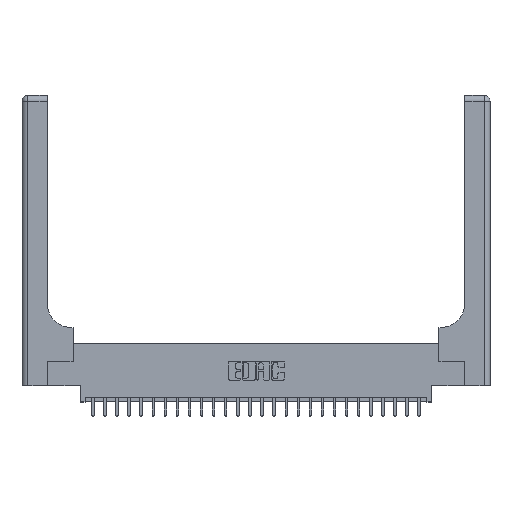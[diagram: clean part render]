
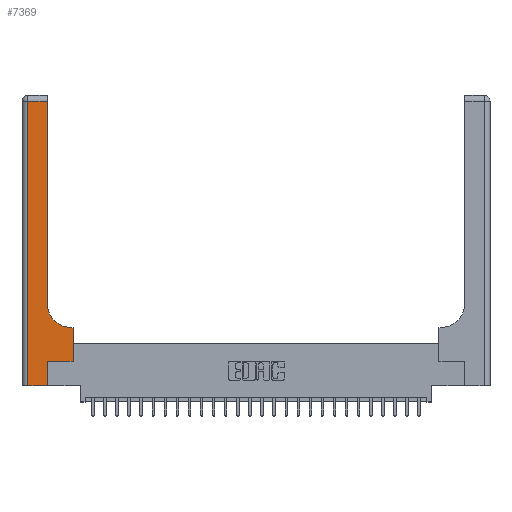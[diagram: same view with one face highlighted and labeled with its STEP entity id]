
A CAD part, top view. The second image highlights one B-rep face of the part: STEP entity #7369.
In plain terms, the highlighted planar face has unit normal (0, 0, 1).
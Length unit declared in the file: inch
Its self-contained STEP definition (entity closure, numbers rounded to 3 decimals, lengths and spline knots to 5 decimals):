
#612 = CARTESIAN_POINT ( 'NONE',  ( 0.26, 2.94, 0.37 ) ) ;
#1178 = LINE ( 'NONE', #20961, #21587 ) ;
#1230 = DIRECTION ( 'NONE',  ( 0., 1., 0. ) ) ;
#1351 = ORIENTED_EDGE ( 'NONE', *, *, #3178, .T. ) ;
#1502 = CARTESIAN_POINT ( 'NONE',  ( 0.265, 0., 0.37 ) ) ;
#1601 = LINE ( 'NONE', #24904, #11589 ) ;
#1966 = CARTESIAN_POINT ( 'NONE',  ( 0., 3., 0.37 ) ) ;
#2355 = CARTESIAN_POINT ( 'NONE',  ( 0.265, 0.25, 0.37 ) ) ;
#3028 = CARTESIAN_POINT ( 'NONE',  ( 0.51, 0.85, 0.37 ) ) ;
#3178 = EDGE_CURVE ( 'NONE', #20229, #8205, #5353, .T. ) ;
#3802 = VERTEX_POINT ( 'NONE', #20566 ) ;
#3982 = DIRECTION ( 'NONE',  ( -1., 0., 0. ) ) ;
#4695 = ORIENTED_EDGE ( 'NONE', *, *, #15627, .T. ) ;
#5033 = DIRECTION ( 'NONE',  ( 1., 0., 0. ) ) ;
#5195 = FACE_OUTER_BOUND ( 'NONE', #14961, .T. ) ;
#5353 = LINE ( 'NONE', #12642, #10020 ) ;
#5553 = CARTESIAN_POINT ( 'NONE',  ( 0.528, 0.25, 0.37 ) ) ;
#6558 = VERTEX_POINT ( 'NONE', #24060 ) ;
#6663 = ORIENTED_EDGE ( 'NONE', *, *, #11526, .T. ) ;
#6752 = DIRECTION ( 'NONE',  ( 0., 1., 0. ) ) ;
#7072 = VERTEX_POINT ( 'NONE', #2355 ) ;
#7360 = ORIENTED_EDGE ( 'NONE', *, *, #19869, .T. ) ;
#7369 = ADVANCED_FACE ( 'NONE', ( #5195 ), #13885, .F. ) ;
#7524 = LINE ( 'NONE', #1502, #14018 ) ;
#7552 = DIRECTION ( 'NONE',  ( 0., 1., 0. ) ) ;
#8205 = VERTEX_POINT ( 'NONE', #13317 ) ;
#8500 = AXIS2_PLACEMENT_3D ( 'NONE', #1966, #15840, #3982 ) ;
#8737 = DIRECTION ( 'NONE',  ( -1., 0., 0. ) ) ;
#9315 = CARTESIAN_POINT ( 'NONE',  ( 0.528, 0.6, 0.37 ) ) ;
#9894 = ORIENTED_EDGE ( 'NONE', *, *, #23457, .T. ) ;
#10020 = VECTOR ( 'NONE', #8737, 39.37008 ) ;
#10706 = EDGE_CURVE ( 'NONE', #22985, #21063, #24483, .T. ) ;
#11335 = LINE ( 'NONE', #19174, #21130 ) ;
#11526 = EDGE_CURVE ( 'NONE', #6558, #15386, #11335, .T. ) ;
#11589 = VECTOR ( 'NONE', #15210, 39.37008 ) ;
#11832 = ORIENTED_EDGE ( 'NONE', *, *, #24746, .T. ) ;
#12306 = ORIENTED_EDGE ( 'NONE', *, *, #20214, .T. ) ;
#12642 = CARTESIAN_POINT ( 'NONE',  ( 0., 2.94, 0.37 ) ) ;
#13317 = CARTESIAN_POINT ( 'NONE',  ( 0.06, 2.94, 0.37 ) ) ;
#13559 = VECTOR ( 'NONE', #24233, 39.37008 ) ;
#13624 = VERTEX_POINT ( 'NONE', #24182 ) ;
#13631 = DIRECTION ( 'NONE',  ( 1., 0., 0. ) ) ;
#13885 = PLANE ( 'NONE',  #8500 ) ;
#14018 = VECTOR ( 'NONE', #7552, 39.37008 ) ;
#14672 = LINE ( 'NONE', #15596, #24397 ) ;
#14961 = EDGE_LOOP ( 'NONE', ( #4695, #1351, #9894, #6663, #7360, #19948, #23907, #12306, #11832 ) ) ;
#15210 = DIRECTION ( 'NONE',  ( 0., -1., 0. ) ) ;
#15386 = VERTEX_POINT ( 'NONE', #21834 ) ;
#15596 = CARTESIAN_POINT ( 'NONE',  ( 0.265, 0.25, 0.37 ) ) ;
#15627 = EDGE_CURVE ( 'NONE', #3802, #20229, #1178, .T. ) ;
#15830 = LINE ( 'NONE', #22298, #13559 ) ;
#15840 = DIRECTION ( 'NONE',  ( 0., 0., -1. ) ) ;
#16859 = DIRECTION ( 'NONE',  ( 0., 0., -1. ) ) ;
#18735 = VECTOR ( 'NONE', #6752, 39.37008 ) ;
#19174 = CARTESIAN_POINT ( 'NONE',  ( 0., 0., 0.37 ) ) ;
#19275 = EDGE_CURVE ( 'NONE', #7072, #22985, #14672, .T. ) ;
#19869 = EDGE_CURVE ( 'NONE', #15386, #7072, #7524, .T. ) ;
#19874 = CIRCLE ( 'NONE', #23030, 0.25 ) ;
#19948 = ORIENTED_EDGE ( 'NONE', *, *, #19275, .T. ) ;
#20214 = EDGE_CURVE ( 'NONE', #21063, #13624, #15830, .T. ) ;
#20229 = VERTEX_POINT ( 'NONE', #612 ) ;
#20566 = CARTESIAN_POINT ( 'NONE',  ( 0.26, 0.85, 0.37 ) ) ;
#20961 = CARTESIAN_POINT ( 'NONE',  ( 0.26, 3., 0.37 ) ) ;
#21063 = VERTEX_POINT ( 'NONE', #9315 ) ;
#21130 = VECTOR ( 'NONE', #21140, 39.37008 ) ;
#21140 = DIRECTION ( 'NONE',  ( 1., 0., 0. ) ) ;
#21587 = VECTOR ( 'NONE', #1230, 39.37008 ) ;
#21834 = CARTESIAN_POINT ( 'NONE',  ( 0.265, 0., 0.37 ) ) ;
#22298 = CARTESIAN_POINT ( 'NONE',  ( 0.26, 0.6, 0.37 ) ) ;
#22372 = CARTESIAN_POINT ( 'NONE',  ( 0.528, 0.25, 0.37 ) ) ;
#22985 = VERTEX_POINT ( 'NONE', #5553 ) ;
#23030 = AXIS2_PLACEMENT_3D ( 'NONE', #3028, #16859, #5033 ) ;
#23457 = EDGE_CURVE ( 'NONE', #8205, #6558, #1601, .T. ) ;
#23907 = ORIENTED_EDGE ( 'NONE', *, *, #10706, .T. ) ;
#24060 = CARTESIAN_POINT ( 'NONE',  ( 0.06, 0., 0.37 ) ) ;
#24182 = CARTESIAN_POINT ( 'NONE',  ( 0.51, 0.6, 0.37 ) ) ;
#24233 = DIRECTION ( 'NONE',  ( -1., 0., 0. ) ) ;
#24397 = VECTOR ( 'NONE', #13631, 39.37008 ) ;
#24483 = LINE ( 'NONE', #22372, #18735 ) ;
#24746 = EDGE_CURVE ( 'NONE', #13624, #3802, #19874, .T. ) ;
#24904 = CARTESIAN_POINT ( 'NONE',  ( 0.06, 3., 0.37 ) ) ;
